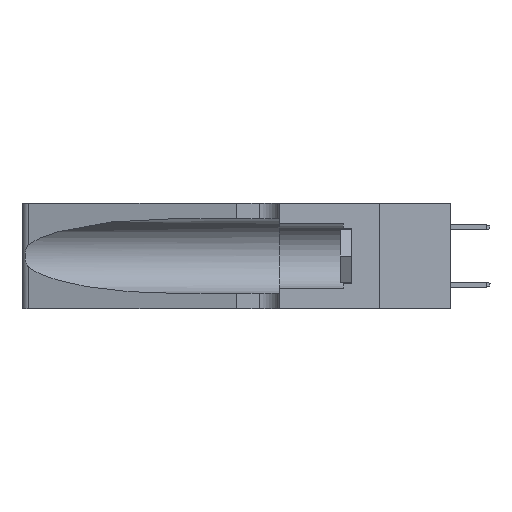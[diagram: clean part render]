
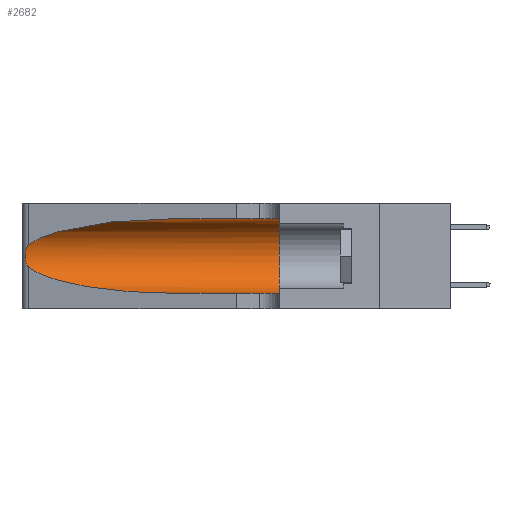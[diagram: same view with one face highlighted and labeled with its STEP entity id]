
A CAD part, left-side view. The second image highlights one B-rep face of the part: STEP entity #2682.
In plain terms, the highlighted cylindrical face has radius 3.308 mm (diameter 6.617 mm), a partial arc.
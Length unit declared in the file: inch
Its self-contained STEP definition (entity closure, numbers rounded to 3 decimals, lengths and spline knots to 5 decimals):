
#1328 = CARTESIAN_POINT ( 'NONE',  ( 0.1305, 0.72297, 0.31525 ) ) ;
#1990 = CARTESIAN_POINT ( 'NONE',  ( 0.1305, 1.61858, 0.31525 ) ) ;
#2467 = DIRECTION ( 'NONE',  ( 0., 0., 1. ) ) ;
#2682 = ADVANCED_FACE ( 'NONE', ( #14813 ), #21869, .F. ) ;
#2746 = CARTESIAN_POINT ( 'NONE',  ( 0.25487, 1.22718, 0.22369 ) ) ;
#4221 = ORIENTED_EDGE ( 'NONE', *, *, #9545, .T. ) ;
#4291 = DIRECTION ( 'NONE',  ( 0., -1., 0. ) ) ;
#5159 = CARTESIAN_POINT ( 'NONE',  ( 0.2373, 1.15595, 0.28018 ) ) ;
#5261 = ORIENTED_EDGE ( 'NONE', *, *, #6733, .T. ) ;
#5299 = VERTEX_POINT ( 'NONE', #7597 ) ;
#5711 = CARTESIAN_POINT ( 'NONE',  ( 0.26075, 1.23896, 0.178 ) ) ;
#5774 = CARTESIAN_POINT ( 'NONE',  ( 0.25487, 1.22718, 0.14631 ) ) ;
#6312 = ORIENTED_EDGE ( 'NONE', *, *, #14694, .T. ) ;
#6733 = EDGE_CURVE ( 'NONE', #7119, #11492, #18306, .T. ) ;
#7109 = CARTESIAN_POINT ( 'NONE',  ( 0.25487, 1.22718, 0.22369 ) ) ;
#7119 = VERTEX_POINT ( 'NONE', #10647 ) ;
#7223 = CARTESIAN_POINT ( 'NONE',  ( 0.25639, 1.23186, 0.15144 ) ) ;
#7293 = AXIS2_PLACEMENT_3D ( 'NONE', #20174, #4291, #12031 ) ;
#7417 = EDGE_CURVE ( 'NONE', #5299, #10301, #13263, .T. ) ;
#7597 = CARTESIAN_POINT ( 'NONE',  ( 0.1305, 0.72297, 0.31525 ) ) ;
#7740 = VECTOR ( 'NONE', #16448, 39.37008 ) ;
#8402 = CARTESIAN_POINT ( 'NONE',  ( 0.1305, 0.35, 0.31525 ) ) ;
#8613 = CARTESIAN_POINT ( 'NONE',  ( 0.2373, 1.15595, 0.08982 ) ) ;
#8803 = B_SPLINE_CURVE_WITH_KNOTS ( 'NONE', 3,
 ( #7109, #10672, #21101, #10436, #8963, #8856, #14268, #5711, #17747, #15887, #9192, #7223, #15990, #12780 ),
 .UNSPECIFIED., .F., .F.,
 ( 4, 2, 2, 2, 2, 2, 4 ),
 ( 0., 0.00027, 0.00053, 0.00107, 0.0016, 0.00187, 0.00214 ),
 .UNSPECIFIED. ) ;
#8856 = CARTESIAN_POINT ( 'NONE',  ( 0.26018, 1.23835, 0.19895 ) ) ;
#8963 = CARTESIAN_POINT ( 'NONE',  ( 0.25854, 1.2359, 0.20912 ) ) ;
#9192 = CARTESIAN_POINT ( 'NONE',  ( 0.25789, 1.23486, 0.15765 ) ) ;
#9418 = LINE ( 'NONE', #1990, #21954 ) ;
#9545 = EDGE_CURVE ( 'NONE', #10385, #7119, #17379, .T. ) ;
#10301 = VERTEX_POINT ( 'NONE', #2746 ) ;
#10385 = VERTEX_POINT ( 'NONE', #5774 ) ;
#10436 = CARTESIAN_POINT ( 'NONE',  ( 0.25787, 1.23484, 0.2124 ) ) ;
#10527 = CARTESIAN_POINT ( 'NONE',  ( 0.25487, 1.22718, 0.14631 ) ) ;
#10647 = CARTESIAN_POINT ( 'NONE',  ( 0.1305, 0.72297, 0.05475 ) ) ;
#10672 = CARTESIAN_POINT ( 'NONE',  ( 0.25555, 1.22994, 0.2215 ) ) ;
#10723 = VERTEX_POINT ( 'NONE', #8402 ) ;
#11492 = VERTEX_POINT ( 'NONE', #19386 ) ;
#11761 = ORIENTED_EDGE ( 'NONE', *, *, #7417, .T. ) ;
#12031 = DIRECTION ( 'NONE',  ( 0., 0., -1. ) ) ;
#12364 = ORIENTED_EDGE ( 'NONE', *, *, #12952, .F. ) ;
#12780 = CARTESIAN_POINT ( 'NONE',  ( 0.25487, 1.22718, 0.14631 ) ) ;
#12952 = EDGE_CURVE ( 'NONE', #10723, #11492, #15222, .T. ) ;
#13085 = ORIENTED_EDGE ( 'NONE', *, *, #17138, .F. ) ;
#13263 =( BOUNDED_CURVE ( )  B_SPLINE_CURVE ( 3, ( #1328, #21014, #5159, #13741 ),
 .UNSPECIFIED., .F., .F. ) 
 B_SPLINE_CURVE_WITH_KNOTS ( ( 4, 4 ),
 ( 1.5708, 2.84003 ),
 .UNSPECIFIED. ) 
 CURVE ( )  GEOMETRIC_REPRESENTATION_ITEM ( )  RATIONAL_B_SPLINE_CURVE ( ( 1., 0.87, 0.87, 1. ) ) 
 REPRESENTATION_ITEM ( '' )  );
#13741 = CARTESIAN_POINT ( 'NONE',  ( 0.25487, 1.22718, 0.22369 ) ) ;
#13802 = CARTESIAN_POINT ( 'NONE',  ( 0.18966, 0.96281, 0.05475 ) ) ;
#14268 = CARTESIAN_POINT ( 'NONE',  ( 0.26075, 1.23896, 0.19203 ) ) ;
#14694 = EDGE_CURVE ( 'NONE', #10301, #10385, #8803, .T. ) ;
#14813 = FACE_OUTER_BOUND ( 'NONE', #17355, .T. ) ;
#15222 = CIRCLE ( 'NONE', #18179, 0.13025 ) ;
#15887 = CARTESIAN_POINT ( 'NONE',  ( 0.25856, 1.23593, 0.16098 ) ) ;
#15990 = CARTESIAN_POINT ( 'NONE',  ( 0.25555, 1.22993, 0.14849 ) ) ;
#16235 = DIRECTION ( 'NONE',  ( 0., -1., 0. ) ) ;
#16448 = DIRECTION ( 'NONE',  ( 0., -1., 0. ) ) ;
#16787 = CARTESIAN_POINT ( 'NONE',  ( 0.1305, 1.61858, 0.05475 ) ) ;
#17138 = EDGE_CURVE ( 'NONE', #5299, #10723, #9418, .T. ) ;
#17355 = EDGE_LOOP ( 'NONE', ( #11761, #6312, #4221, #5261, #12364, #13085 ) ) ;
#17379 =( BOUNDED_CURVE ( )  B_SPLINE_CURVE ( 3, ( #10527, #8613, #13802, #20855 ),
 .UNSPECIFIED., .F., .F. ) 
 B_SPLINE_CURVE_WITH_KNOTS ( ( 4, 4 ),
 ( 3.44316, 4.71239 ),
 .UNSPECIFIED. ) 
 CURVE ( )  GEOMETRIC_REPRESENTATION_ITEM ( )  RATIONAL_B_SPLINE_CURVE ( ( 1., 0.87, 0.87, 1. ) ) 
 REPRESENTATION_ITEM ( '' )  );
#17747 = CARTESIAN_POINT ( 'NONE',  ( 0.26017, 1.23833, 0.17102 ) ) ;
#18179 = AXIS2_PLACEMENT_3D ( 'NONE', #21222, #18573, #2467 ) ;
#18306 = LINE ( 'NONE', #16787, #7740 ) ;
#18573 = DIRECTION ( 'NONE',  ( 0., 1., 0. ) ) ;
#19386 = CARTESIAN_POINT ( 'NONE',  ( 0.1305, 0.35, 0.05475 ) ) ;
#20174 = CARTESIAN_POINT ( 'NONE',  ( 0.1305, 1.61858, 0.185 ) ) ;
#20855 = CARTESIAN_POINT ( 'NONE',  ( 0.1305, 0.72297, 0.05475 ) ) ;
#21014 = CARTESIAN_POINT ( 'NONE',  ( 0.18966, 0.96281, 0.31525 ) ) ;
#21101 = CARTESIAN_POINT ( 'NONE',  ( 0.25639, 1.23184, 0.21858 ) ) ;
#21222 = CARTESIAN_POINT ( 'NONE',  ( 0.1305, 0.35, 0.185 ) ) ;
#21869 = CYLINDRICAL_SURFACE ( 'NONE', #7293, 0.13025 ) ;
#21954 = VECTOR ( 'NONE', #16235, 39.37008 ) ;
